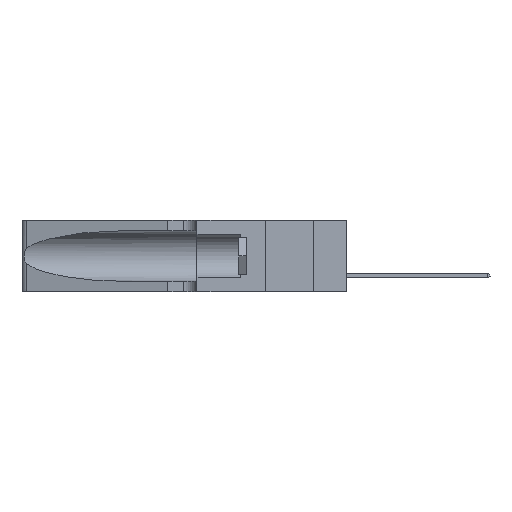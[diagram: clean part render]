
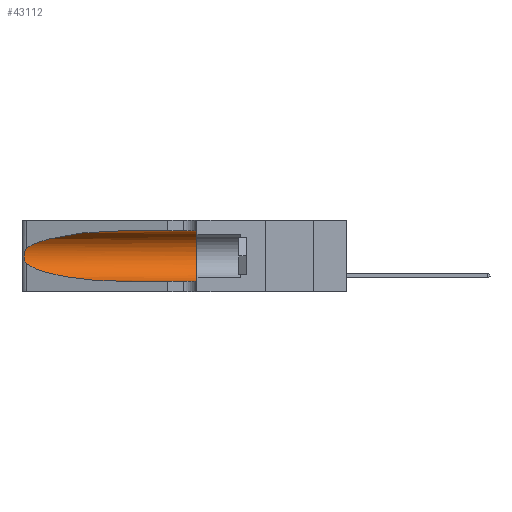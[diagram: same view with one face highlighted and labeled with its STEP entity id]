
A CAD part, left-side view. The second image highlights one B-rep face of the part: STEP entity #43112.
In plain terms, the highlighted cylindrical face has radius 3.308 mm (diameter 6.617 mm), a partial arc.
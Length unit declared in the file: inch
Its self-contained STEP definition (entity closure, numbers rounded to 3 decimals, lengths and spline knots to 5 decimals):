
#2109 = CARTESIAN_POINT ( 'NONE',  ( 0.1305, 0.72297, 0.31525 ) ) ;
#3013 = VERTEX_POINT ( 'NONE', #20064 ) ;
#4143 = B_SPLINE_CURVE_WITH_KNOTS ( 'NONE', 3,
 ( #40225, #39913, #32891, #43804, #47879, #14447, #47726, #47568, #43473, #29035, #32460, #36166, #36626, #33051 ),
 .UNSPECIFIED., .F., .F.,
 ( 4, 2, 2, 2, 2, 2, 4 ),
 ( 0., 0.00027, 0.00053, 0.00107, 0.0016, 0.00187, 0.00214 ),
 .UNSPECIFIED. ) ;
#5081 = CYLINDRICAL_SURFACE ( 'NONE', #8083, 0.13025 ) ;
#6773 = DIRECTION ( 'NONE',  ( 0., 1., 0. ) ) ;
#7311 = CARTESIAN_POINT ( 'NONE',  ( 0.18966, 0.96281, 0.05475 ) ) ;
#7846 = VERTEX_POINT ( 'NONE', #24728 ) ;
#8083 = AXIS2_PLACEMENT_3D ( 'NONE', #16629, #34916, #42712 ) ;
#8911 = EDGE_CURVE ( 'NONE', #39467, #3013, #31061, .T. ) ;
#10347 = ORIENTED_EDGE ( 'NONE', *, *, #8911, .T. ) ;
#12106 = CARTESIAN_POINT ( 'NONE',  ( 0.1305, 1.61858, 0.05475 ) ) ;
#12405 = EDGE_LOOP ( 'NONE', ( #14672, #42028, #13840, #10347, #47880, #46598 ) ) ;
#13433 =( BOUNDED_CURVE ( )  B_SPLINE_CURVE ( 3, ( #36983, #22560, #7311, #44476 ),
 .UNSPECIFIED., .F., .T. ) 
 B_SPLINE_CURVE_WITH_KNOTS ( ( 4, 4 ),
 ( 3.44316, 4.71239 ),
 .UNSPECIFIED. ) 
 CURVE ( )  GEOMETRIC_REPRESENTATION_ITEM ( )  RATIONAL_B_SPLINE_CURVE ( ( 1., 0.87, 0.87, 1. ) ) 
 REPRESENTATION_ITEM ( '' )  );
#13456 = EDGE_CURVE ( 'NONE', #45671, #7846, #30389, .T. ) ;
#13840 = ORIENTED_EDGE ( 'NONE', *, *, #31794, .T. ) ;
#14447 = CARTESIAN_POINT ( 'NONE',  ( 0.26018, 1.23835, 0.19895 ) ) ;
#14672 = ORIENTED_EDGE ( 'NONE', *, *, #28607, .T. ) ;
#16629 = CARTESIAN_POINT ( 'NONE',  ( 0.1305, 1.61858, 0.185 ) ) ;
#18351 = VECTOR ( 'NONE', #45556, 39.37008 ) ;
#20064 = CARTESIAN_POINT ( 'NONE',  ( 0.1305, 0.35, 0.05475 ) ) ;
#20383 = VERTEX_POINT ( 'NONE', #41267 ) ;
#20644 = CARTESIAN_POINT ( 'NONE',  ( 0.2373, 1.15595, 0.28018 ) ) ;
#21428 = CARTESIAN_POINT ( 'NONE',  ( 0.1305, 1.61858, 0.31525 ) ) ;
#22560 = CARTESIAN_POINT ( 'NONE',  ( 0.2373, 1.15595, 0.08982 ) ) ;
#22675 = CARTESIAN_POINT ( 'NONE',  ( 0.25487, 1.22718, 0.14631 ) ) ;
#24728 = CARTESIAN_POINT ( 'NONE',  ( 0.1305, 0.35, 0.31525 ) ) ;
#24963 = DIRECTION ( 'NONE',  ( 0., -1., 0. ) ) ;
#25034 =( BOUNDED_CURVE ( )  B_SPLINE_CURVE ( 3, ( #2109, #46285, #20644, #46606 ),
 .UNSPECIFIED., .F., .T. ) 
 B_SPLINE_CURVE_WITH_KNOTS ( ( 4, 4 ),
 ( 1.5708, 2.84003 ),
 .UNSPECIFIED. ) 
 CURVE ( )  GEOMETRIC_REPRESENTATION_ITEM ( )  RATIONAL_B_SPLINE_CURVE ( ( 1., 0.87, 0.87, 1. ) ) 
 REPRESENTATION_ITEM ( '' )  );
#26508 = CARTESIAN_POINT ( 'NONE',  ( 0.1305, 0.72297, 0.05475 ) ) ;
#28607 = EDGE_CURVE ( 'NONE', #45671, #20383, #25034, .T. ) ;
#28739 = EDGE_CURVE ( 'NONE', #7846, #3013, #37728, .T. ) ;
#29035 = CARTESIAN_POINT ( 'NONE',  ( 0.25856, 1.23593, 0.16098 ) ) ;
#29347 = DIRECTION ( 'NONE',  ( 0., 0., 1. ) ) ;
#30071 = FACE_OUTER_BOUND ( 'NONE', #12405, .T. ) ;
#30389 = LINE ( 'NONE', #21428, #32723 ) ;
#31061 = LINE ( 'NONE', #12106, #18351 ) ;
#31794 = EDGE_CURVE ( 'NONE', #46941, #39467, #13433, .T. ) ;
#32460 = CARTESIAN_POINT ( 'NONE',  ( 0.25789, 1.23486, 0.15765 ) ) ;
#32723 = VECTOR ( 'NONE', #24963, 39.37008 ) ;
#32891 = CARTESIAN_POINT ( 'NONE',  ( 0.25639, 1.23184, 0.21858 ) ) ;
#33051 = CARTESIAN_POINT ( 'NONE',  ( 0.25487, 1.22718, 0.14631 ) ) ;
#34916 = DIRECTION ( 'NONE',  ( 0., -1., 0. ) ) ;
#36166 = CARTESIAN_POINT ( 'NONE',  ( 0.25639, 1.23186, 0.15144 ) ) ;
#36626 = CARTESIAN_POINT ( 'NONE',  ( 0.25555, 1.22993, 0.14849 ) ) ;
#36983 = CARTESIAN_POINT ( 'NONE',  ( 0.25487, 1.22718, 0.14631 ) ) ;
#37728 = CIRCLE ( 'NONE', #45343, 0.13025 ) ;
#39467 = VERTEX_POINT ( 'NONE', #26508 ) ;
#39913 = CARTESIAN_POINT ( 'NONE',  ( 0.25555, 1.22994, 0.2215 ) ) ;
#40225 = CARTESIAN_POINT ( 'NONE',  ( 0.25487, 1.22718, 0.22369 ) ) ;
#40389 = CARTESIAN_POINT ( 'NONE',  ( 0.1305, 0.35, 0.185 ) ) ;
#41267 = CARTESIAN_POINT ( 'NONE',  ( 0.25487, 1.22718, 0.22369 ) ) ;
#42028 = ORIENTED_EDGE ( 'NONE', *, *, #42087, .T. ) ;
#42087 = EDGE_CURVE ( 'NONE', #20383, #46941, #4143, .T. ) ;
#42712 = DIRECTION ( 'NONE',  ( 0., 0., -1. ) ) ;
#43112 = ADVANCED_FACE ( 'NONE', ( #30071 ), #5081, .F. ) ;
#43473 = CARTESIAN_POINT ( 'NONE',  ( 0.26017, 1.23833, 0.17102 ) ) ;
#43804 = CARTESIAN_POINT ( 'NONE',  ( 0.25787, 1.23484, 0.2124 ) ) ;
#44476 = CARTESIAN_POINT ( 'NONE',  ( 0.1305, 0.72297, 0.05475 ) ) ;
#45202 = CARTESIAN_POINT ( 'NONE',  ( 0.1305, 0.72297, 0.31525 ) ) ;
#45343 = AXIS2_PLACEMENT_3D ( 'NONE', #40389, #6773, #29347 ) ;
#45556 = DIRECTION ( 'NONE',  ( 0., -1., 0. ) ) ;
#45671 = VERTEX_POINT ( 'NONE', #45202 ) ;
#46285 = CARTESIAN_POINT ( 'NONE',  ( 0.18966, 0.96281, 0.31525 ) ) ;
#46598 = ORIENTED_EDGE ( 'NONE', *, *, #13456, .F. ) ;
#46606 = CARTESIAN_POINT ( 'NONE',  ( 0.25487, 1.22718, 0.22369 ) ) ;
#46941 = VERTEX_POINT ( 'NONE', #22675 ) ;
#47568 = CARTESIAN_POINT ( 'NONE',  ( 0.26075, 1.23896, 0.178 ) ) ;
#47726 = CARTESIAN_POINT ( 'NONE',  ( 0.26075, 1.23896, 0.19203 ) ) ;
#47879 = CARTESIAN_POINT ( 'NONE',  ( 0.25854, 1.2359, 0.20912 ) ) ;
#47880 = ORIENTED_EDGE ( 'NONE', *, *, #28739, .F. ) ;
